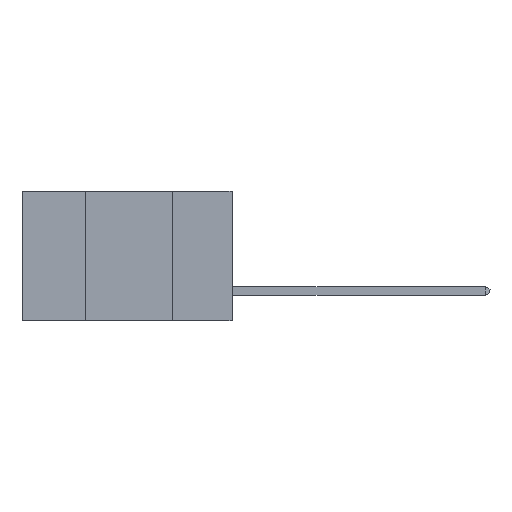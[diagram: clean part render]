
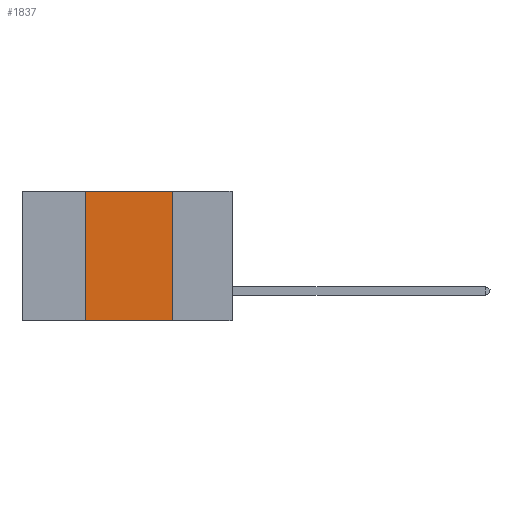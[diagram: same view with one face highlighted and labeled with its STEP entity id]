
A CAD part, left-side view. The second image highlights one B-rep face of the part: STEP entity #1837.
In plain terms, the highlighted planar face has unit normal (-1, 0, 0).
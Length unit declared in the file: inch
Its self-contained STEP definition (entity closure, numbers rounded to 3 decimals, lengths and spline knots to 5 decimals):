
#304 = EDGE_CURVE ( 'NONE', #2974, #3398, #11493, .T. ) ;
#482 = LINE ( 'NONE', #2661, #9405 ) ;
#934 = DIRECTION ( 'NONE',  ( 0., 0., -1. ) ) ;
#1529 = VERTEX_POINT ( 'NONE', #2576 ) ;
#1837 = ADVANCED_FACE ( 'NONE', ( #3854 ), #14430, .F. ) ;
#1854 = LINE ( 'NONE', #7816, #12755 ) ;
#2576 = CARTESIAN_POINT ( 'NONE',  ( 0., 0.17, 0. ) ) ;
#2661 = CARTESIAN_POINT ( 'NONE',  ( 0., 0.6, -0.37 ) ) ;
#2974 = VERTEX_POINT ( 'NONE', #6452 ) ;
#3104 = CARTESIAN_POINT ( 'NONE',  ( 0., 0.17, 0. ) ) ;
#3219 = EDGE_CURVE ( 'NONE', #1529, #5316, #10384, .T. ) ;
#3301 = EDGE_CURVE ( 'NONE', #3398, #1529, #1854, .T. ) ;
#3398 = VERTEX_POINT ( 'NONE', #13980 ) ;
#3854 = FACE_OUTER_BOUND ( 'NONE', #11830, .T. ) ;
#3876 = ORIENTED_EDGE ( 'NONE', *, *, #3219, .F. ) ;
#4013 = AXIS2_PLACEMENT_3D ( 'NONE', #8656, #7532, #7427 ) ;
#4977 = DIRECTION ( 'NONE',  ( 0., -1., 0. ) ) ;
#5316 = VERTEX_POINT ( 'NONE', #5715 ) ;
#5715 = CARTESIAN_POINT ( 'NONE',  ( 0., 0.17, -0.37 ) ) ;
#5932 = ORIENTED_EDGE ( 'NONE', *, *, #11480, .T. ) ;
#6375 = VECTOR ( 'NONE', #934, 39.37008 ) ;
#6452 = CARTESIAN_POINT ( 'NONE',  ( 0., 0.42, -0.37 ) ) ;
#6722 = DIRECTION ( 'NONE',  ( 0., 0., 1. ) ) ;
#7427 = DIRECTION ( 'NONE',  ( 0., 0., -1. ) ) ;
#7532 = DIRECTION ( 'NONE',  ( 1., 0., 0. ) ) ;
#7816 = CARTESIAN_POINT ( 'NONE',  ( 0., 0.6, 0. ) ) ;
#8363 = ORIENTED_EDGE ( 'NONE', *, *, #3301, .F. ) ;
#8656 = CARTESIAN_POINT ( 'NONE',  ( 0., 0.6, 0. ) ) ;
#9340 = VECTOR ( 'NONE', #6722, 39.37008 ) ;
#9405 = VECTOR ( 'NONE', #4977, 39.37008 ) ;
#10384 = LINE ( 'NONE', #3104, #6375 ) ;
#11326 = DIRECTION ( 'NONE',  ( 0., -1., 0. ) ) ;
#11480 = EDGE_CURVE ( 'NONE', #2974, #5316, #482, .T. ) ;
#11493 = LINE ( 'NONE', #15011, #9340 ) ;
#11830 = EDGE_LOOP ( 'NONE', ( #3876, #8363, #12573, #5932 ) ) ;
#12573 = ORIENTED_EDGE ( 'NONE', *, *, #304, .F. ) ;
#12755 = VECTOR ( 'NONE', #11326, 39.37008 ) ;
#13980 = CARTESIAN_POINT ( 'NONE',  ( 0., 0.42, 0. ) ) ;
#14430 = PLANE ( 'NONE',  #4013 ) ;
#15011 = CARTESIAN_POINT ( 'NONE',  ( 0., 0.42, 0. ) ) ;
